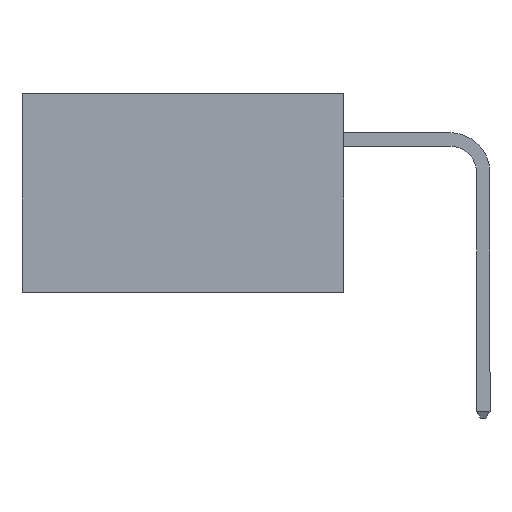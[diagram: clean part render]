
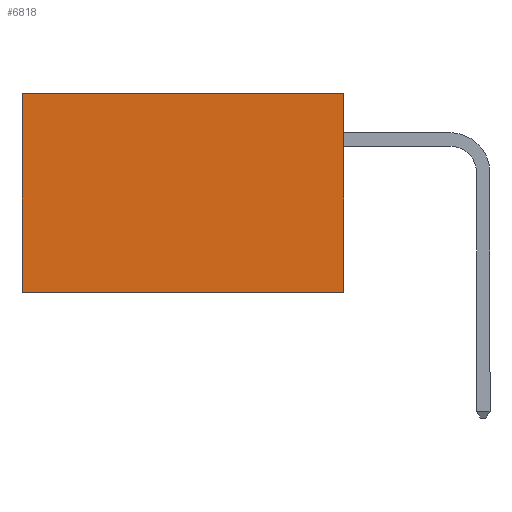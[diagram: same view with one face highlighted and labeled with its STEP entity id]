
A CAD part, left-side view. The second image highlights one B-rep face of the part: STEP entity #6818.
In plain terms, the highlighted planar face has unit normal (-1, 0, 0).
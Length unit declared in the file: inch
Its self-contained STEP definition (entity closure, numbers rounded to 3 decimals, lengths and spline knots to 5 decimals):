
#657 = EDGE_CURVE ( 'NONE', #4408, #8032, #2413, .T. ) ;
#776 = FACE_OUTER_BOUND ( 'NONE', #5800, .T. ) ;
#938 = AXIS2_PLACEMENT_3D ( 'NONE', #5293, #4014, #7787 ) ;
#1101 = CARTESIAN_POINT ( 'NONE',  ( 0.2615, 0., -0.37 ) ) ;
#1116 = VECTOR ( 'NONE', #1756, 39.37008 ) ;
#1119 = EDGE_CURVE ( 'NONE', #4408, #1524, #7303, .T. ) ;
#1524 = VERTEX_POINT ( 'NONE', #1101 ) ;
#1756 = DIRECTION ( 'NONE',  ( 0., 0., -1. ) ) ;
#2172 = LINE ( 'NONE', #3918, #7241 ) ;
#2284 = DIRECTION ( 'NONE',  ( 0., 1., 0. ) ) ;
#2413 = LINE ( 'NONE', #4884, #4150 ) ;
#2709 = LINE ( 'NONE', #4302, #4466 ) ;
#2749 = DIRECTION ( 'NONE',  ( 0., 0., -1. ) ) ;
#3008 = ORIENTED_EDGE ( 'NONE', *, *, #1119, .F. ) ;
#3211 = EDGE_CURVE ( 'NONE', #1524, #6358, #2172, .T. ) ;
#3455 = DIRECTION ( 'NONE',  ( 0., 1., 0. ) ) ;
#3489 = CARTESIAN_POINT ( 'NONE',  ( 0.2615, 0.6, 0. ) ) ;
#3918 = CARTESIAN_POINT ( 'NONE',  ( 0.2615, 0., -0.37 ) ) ;
#4014 = DIRECTION ( 'NONE',  ( 1., 0., 0. ) ) ;
#4150 = VECTOR ( 'NONE', #2284, 39.37008 ) ;
#4279 = EDGE_CURVE ( 'NONE', #8032, #6358, #2709, .T. ) ;
#4302 = CARTESIAN_POINT ( 'NONE',  ( 0.2615, 0.6, -0.37 ) ) ;
#4408 = VERTEX_POINT ( 'NONE', #5009 ) ;
#4466 = VECTOR ( 'NONE', #2749, 39.37008 ) ;
#4468 = CARTESIAN_POINT ( 'NONE',  ( 0.2615, 0.6, -0.37 ) ) ;
#4884 = CARTESIAN_POINT ( 'NONE',  ( 0.2615, 0., 0. ) ) ;
#5009 = CARTESIAN_POINT ( 'NONE',  ( 0.2615, 0., 0. ) ) ;
#5293 = CARTESIAN_POINT ( 'NONE',  ( 0.2615, 0., -0.37 ) ) ;
#5800 = EDGE_LOOP ( 'NONE', ( #7131, #6986, #3008, #6947 ) ) ;
#6358 = VERTEX_POINT ( 'NONE', #4468 ) ;
#6546 = PLANE ( 'NONE',  #938 ) ;
#6818 = ADVANCED_FACE ( 'NONE', ( #776 ), #6546, .F. ) ;
#6947 = ORIENTED_EDGE ( 'NONE', *, *, #657, .T. ) ;
#6986 = ORIENTED_EDGE ( 'NONE', *, *, #3211, .F. ) ;
#7131 = ORIENTED_EDGE ( 'NONE', *, *, #4279, .T. ) ;
#7241 = VECTOR ( 'NONE', #3455, 39.37008 ) ;
#7303 = LINE ( 'NONE', #7438, #1116 ) ;
#7438 = CARTESIAN_POINT ( 'NONE',  ( 0.2615, 0., -0.37 ) ) ;
#7787 = DIRECTION ( 'NONE',  ( 0., 0., -1. ) ) ;
#8032 = VERTEX_POINT ( 'NONE', #3489 ) ;
